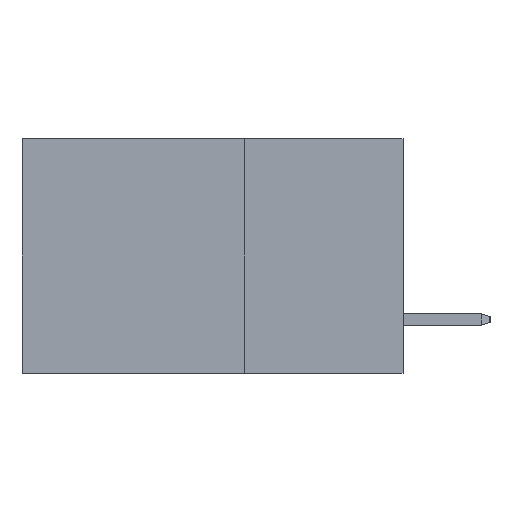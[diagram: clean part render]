
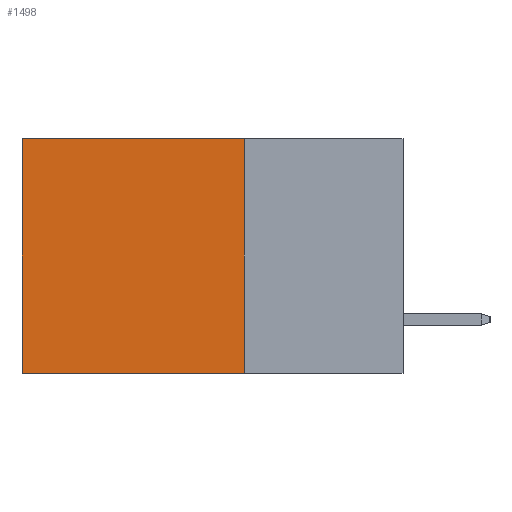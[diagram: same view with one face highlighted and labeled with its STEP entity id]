
A CAD part, left-side view. The second image highlights one B-rep face of the part: STEP entity #1498.
In plain terms, the highlighted planar face has unit normal (-1, 0, 0).
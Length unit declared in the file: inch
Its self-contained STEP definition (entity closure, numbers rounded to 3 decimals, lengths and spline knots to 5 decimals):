
#258 = DIRECTION ( 'NONE',  ( 0., 1., 0. ) ) ;
#334 = EDGE_LOOP ( 'NONE', ( #2986, #8661, #777, #4164 ) ) ;
#403 = LINE ( 'NONE', #1213, #8685 ) ;
#557 = CARTESIAN_POINT ( 'NONE',  ( 0.2875, 0.6, -0.37 ) ) ;
#717 = VECTOR ( 'NONE', #8721, 39.37008 ) ;
#726 = CARTESIAN_POINT ( 'NONE',  ( 0.2875, 0.25, 0. ) ) ;
#769 = CARTESIAN_POINT ( 'NONE',  ( 0.2875, 0.25, 0. ) ) ;
#777 = ORIENTED_EDGE ( 'NONE', *, *, #1220, .F. ) ;
#1213 = CARTESIAN_POINT ( 'NONE',  ( 0.2875, 0.25, 0. ) ) ;
#1220 = EDGE_CURVE ( 'NONE', #7400, #1297, #3074, .T. ) ;
#1297 = VERTEX_POINT ( 'NONE', #5181 ) ;
#1498 = ADVANCED_FACE ( 'NONE', ( #8077 ), #6097, .F. ) ;
#2986 = ORIENTED_EDGE ( 'NONE', *, *, #6847, .T. ) ;
#3074 = LINE ( 'NONE', #726, #717 ) ;
#3486 = CARTESIAN_POINT ( 'NONE',  ( 0.2875, 0.6, 0. ) ) ;
#3651 = VERTEX_POINT ( 'NONE', #3486 ) ;
#4164 = ORIENTED_EDGE ( 'NONE', *, *, #8636, .T. ) ;
#4207 = DIRECTION ( 'NONE',  ( 0., 0., -1. ) ) ;
#5181 = CARTESIAN_POINT ( 'NONE',  ( 0.2875, 0.25, -0.37 ) ) ;
#5498 = LINE ( 'NONE', #6211, #8041 ) ;
#5701 = CARTESIAN_POINT ( 'NONE',  ( 0.2875, 0.25, 0. ) ) ;
#6097 = PLANE ( 'NONE',  #8832 ) ;
#6211 = CARTESIAN_POINT ( 'NONE',  ( 0.2875, 0.6, 0. ) ) ;
#6814 = CARTESIAN_POINT ( 'NONE',  ( 0.2875, 0.25, -0.37 ) ) ;
#6847 = EDGE_CURVE ( 'NONE', #3651, #8146, #5498, .T. ) ;
#6932 = DIRECTION ( 'NONE',  ( 0., 0., -1. ) ) ;
#7233 = DIRECTION ( 'NONE',  ( 1., 0., 0. ) ) ;
#7400 = VERTEX_POINT ( 'NONE', #769 ) ;
#8041 = VECTOR ( 'NONE', #6932, 39.37008 ) ;
#8077 = FACE_OUTER_BOUND ( 'NONE', #334, .T. ) ;
#8143 = LINE ( 'NONE', #6814, #8517 ) ;
#8146 = VERTEX_POINT ( 'NONE', #557 ) ;
#8517 = VECTOR ( 'NONE', #258, 39.37008 ) ;
#8636 = EDGE_CURVE ( 'NONE', #7400, #3651, #403, .T. ) ;
#8661 = ORIENTED_EDGE ( 'NONE', *, *, #8930, .F. ) ;
#8685 = VECTOR ( 'NONE', #9200, 39.37008 ) ;
#8721 = DIRECTION ( 'NONE',  ( 0., 0., -1. ) ) ;
#8832 = AXIS2_PLACEMENT_3D ( 'NONE', #5701, #7233, #4207 ) ;
#8930 = EDGE_CURVE ( 'NONE', #1297, #8146, #8143, .T. ) ;
#9200 = DIRECTION ( 'NONE',  ( 0., 1., 0. ) ) ;
